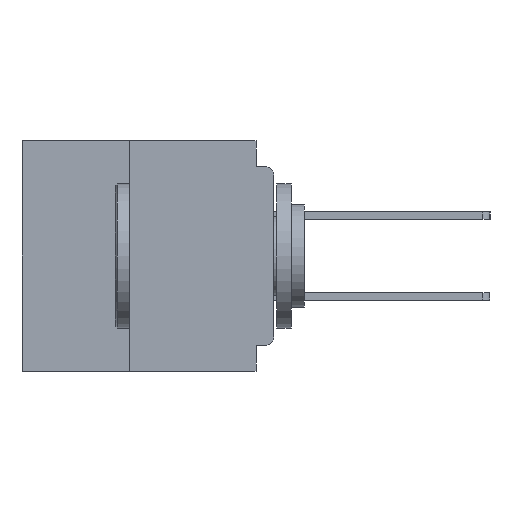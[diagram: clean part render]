
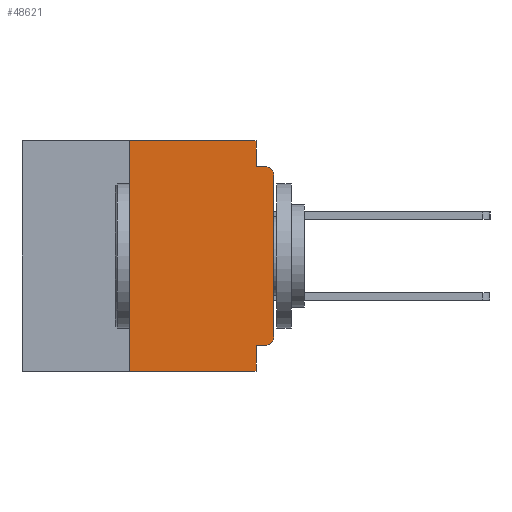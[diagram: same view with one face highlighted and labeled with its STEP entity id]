
A CAD part, left-side view. The second image highlights one B-rep face of the part: STEP entity #48621.
In plain terms, the highlighted planar face has unit normal (-1, 0, 0).
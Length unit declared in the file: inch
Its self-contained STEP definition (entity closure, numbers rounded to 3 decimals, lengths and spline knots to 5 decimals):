
#905 = EDGE_CURVE ( 'NONE', #17620, #8315, #34957, .T. ) ;
#985 = VECTOR ( 'NONE', #28953, 39.37008 ) ;
#2715 = DIRECTION ( 'NONE',  ( 0., 0., 1. ) ) ;
#2888 = VERTEX_POINT ( 'NONE', #24650 ) ;
#4679 = CARTESIAN_POINT ( 'NONE',  ( 0., 0., -0.355 ) ) ;
#5258 = LINE ( 'NONE', #41412, #15581 ) ;
#5290 = ORIENTED_EDGE ( 'NONE', *, *, #15319, .F. ) ;
#6650 = LINE ( 'NONE', #43090, #39235 ) ;
#7135 = ORIENTED_EDGE ( 'NONE', *, *, #19548, .F. ) ;
#8011 = AXIS2_PLACEMENT_3D ( 'NONE', #48919, #22522, #53294 ) ;
#8315 = VERTEX_POINT ( 'NONE', #11666 ) ;
#8760 = CARTESIAN_POINT ( 'NONE',  ( 0., 0., -0.06 ) ) ;
#9003 = EDGE_CURVE ( 'NONE', #41729, #29477, #6650, .T. ) ;
#9111 = DIRECTION ( 'NONE',  ( 0., 1., 0. ) ) ;
#11666 = CARTESIAN_POINT ( 'NONE',  ( 0., 0.031, -0.045 ) ) ;
#11951 = PLANE ( 'NONE',  #46268 ) ;
#12062 = EDGE_CURVE ( 'NONE', #35264, #17620, #5258, .T. ) ;
#12075 = ORIENTED_EDGE ( 'NONE', *, *, #16213, .T. ) ;
#14501 = VERTEX_POINT ( 'NONE', #50160 ) ;
#14822 = DIRECTION ( 'NONE',  ( 0., -1., 0. ) ) ;
#14839 = DIRECTION ( 'NONE',  ( 0., -1., 0. ) ) ;
#15319 = EDGE_CURVE ( 'NONE', #14501, #35264, #21552, .T. ) ;
#15581 = VECTOR ( 'NONE', #14839, 39.37008 ) ;
#15709 = DIRECTION ( 'NONE',  ( 0., 0., 1. ) ) ;
#15970 = EDGE_CURVE ( 'NONE', #43881, #25812, #56181, .T. ) ;
#16213 = EDGE_CURVE ( 'NONE', #50060, #43881, #20297, .T. ) ;
#16658 = DIRECTION ( 'NONE',  ( 0., -1., 0. ) ) ;
#17554 = CARTESIAN_POINT ( 'NONE',  ( 0., 0.031, 0. ) ) ;
#17620 = VERTEX_POINT ( 'NONE', #49632 ) ;
#17818 = ORIENTED_EDGE ( 'NONE', *, *, #25646, .T. ) ;
#19438 = ORIENTED_EDGE ( 'NONE', *, *, #31603, .T. ) ;
#19548 = EDGE_CURVE ( 'NONE', #8315, #2888, #42759, .T. ) ;
#20297 = CIRCLE ( 'NONE', #8011, 0.015 ) ;
#20922 = DIRECTION ( 'NONE',  ( 0., 0., -1. ) ) ;
#20997 = CARTESIAN_POINT ( 'NONE',  ( 0., 0.015, -0.355 ) ) ;
#21552 = LINE ( 'NONE', #42319, #33301 ) ;
#22522 = DIRECTION ( 'NONE',  ( -1., 0., 0. ) ) ;
#22762 = EDGE_CURVE ( 'NONE', #50060, #41729, #37010, .T. ) ;
#23556 = CARTESIAN_POINT ( 'NONE',  ( 0., 0.015, -0.06 ) ) ;
#23901 = VECTOR ( 'NONE', #9111, 39.37008 ) ;
#24650 = CARTESIAN_POINT ( 'NONE',  ( 0., 0.015, -0.045 ) ) ;
#24797 = CIRCLE ( 'NONE', #45091, 0.015 ) ;
#25646 = EDGE_CURVE ( 'NONE', #14501, #29477, #37342, .T. ) ;
#25812 = VERTEX_POINT ( 'NONE', #8760 ) ;
#28032 = DIRECTION ( 'NONE',  ( 0., 0., -1. ) ) ;
#28715 = ORIENTED_EDGE ( 'NONE', *, *, #22762, .F. ) ;
#28953 = DIRECTION ( 'NONE',  ( 0., 0., -1. ) ) ;
#29477 = VERTEX_POINT ( 'NONE', #39178 ) ;
#31022 = VECTOR ( 'NONE', #14822, 39.37008 ) ;
#31603 = EDGE_CURVE ( 'NONE', #25812, #2888, #24797, .T. ) ;
#33301 = VECTOR ( 'NONE', #15709, 39.37008 ) ;
#34363 = ORIENTED_EDGE ( 'NONE', *, *, #905, .F. ) ;
#34815 = CARTESIAN_POINT ( 'NONE',  ( 0., 0.25, 0. ) ) ;
#34957 = LINE ( 'NONE', #17554, #985 ) ;
#35264 = VERTEX_POINT ( 'NONE', #34815 ) ;
#36945 = CARTESIAN_POINT ( 'NONE',  ( 0., 0., -0.045 ) ) ;
#37010 = LINE ( 'NONE', #4679, #23901 ) ;
#37342 = LINE ( 'NONE', #38799, #47693 ) ;
#38321 = CARTESIAN_POINT ( 'NONE',  ( 0., 0.437, 0. ) ) ;
#38799 = CARTESIAN_POINT ( 'NONE',  ( 0., 0.437, -0.4 ) ) ;
#39178 = CARTESIAN_POINT ( 'NONE',  ( 0., 0.031, -0.4 ) ) ;
#39235 = VECTOR ( 'NONE', #51873, 39.37008 ) ;
#40866 = ORIENTED_EDGE ( 'NONE', *, *, #9003, .F. ) ;
#41412 = CARTESIAN_POINT ( 'NONE',  ( 0., 0.437, 0. ) ) ;
#41729 = VERTEX_POINT ( 'NONE', #50642 ) ;
#42319 = CARTESIAN_POINT ( 'NONE',  ( 0., 0.25, -0.4 ) ) ;
#42759 = LINE ( 'NONE', #36945, #31022 ) ;
#43090 = CARTESIAN_POINT ( 'NONE',  ( 0., 0.031, -0.4 ) ) ;
#43881 = VERTEX_POINT ( 'NONE', #56388 ) ;
#44582 = VECTOR ( 'NONE', #2715, 39.37008 ) ;
#45091 = AXIS2_PLACEMENT_3D ( 'NONE', #23556, #54304, #28032 ) ;
#45723 = ORIENTED_EDGE ( 'NONE', *, *, #12062, .F. ) ;
#46268 = AXIS2_PLACEMENT_3D ( 'NONE', #38321, #47383, #20922 ) ;
#47123 = EDGE_LOOP ( 'NONE', ( #55165, #19438, #7135, #34363, #45723, #5290, #17818, #40866, #28715, #12075 ) ) ;
#47383 = DIRECTION ( 'NONE',  ( 1., 0., 0. ) ) ;
#47693 = VECTOR ( 'NONE', #16658, 39.37008 ) ;
#48621 = ADVANCED_FACE ( 'NONE', ( #48790 ), #11951, .F. ) ;
#48790 = FACE_OUTER_BOUND ( 'NONE', #47123, .T. ) ;
#48919 = CARTESIAN_POINT ( 'NONE',  ( 0., 0.015, -0.34 ) ) ;
#49632 = CARTESIAN_POINT ( 'NONE',  ( 0., 0.031, 0. ) ) ;
#50060 = VERTEX_POINT ( 'NONE', #20997 ) ;
#50160 = CARTESIAN_POINT ( 'NONE',  ( 0., 0.25, -0.4 ) ) ;
#50642 = CARTESIAN_POINT ( 'NONE',  ( 0., 0.031, -0.355 ) ) ;
#51221 = CARTESIAN_POINT ( 'NONE',  ( 0., 0., 0. ) ) ;
#51873 = DIRECTION ( 'NONE',  ( 0., 0., -1. ) ) ;
#53294 = DIRECTION ( 'NONE',  ( 0., 0., -1. ) ) ;
#54304 = DIRECTION ( 'NONE',  ( -1., 0., 0. ) ) ;
#55165 = ORIENTED_EDGE ( 'NONE', *, *, #15970, .T. ) ;
#56181 = LINE ( 'NONE', #51221, #44582 ) ;
#56388 = CARTESIAN_POINT ( 'NONE',  ( 0., 0., -0.34 ) ) ;
